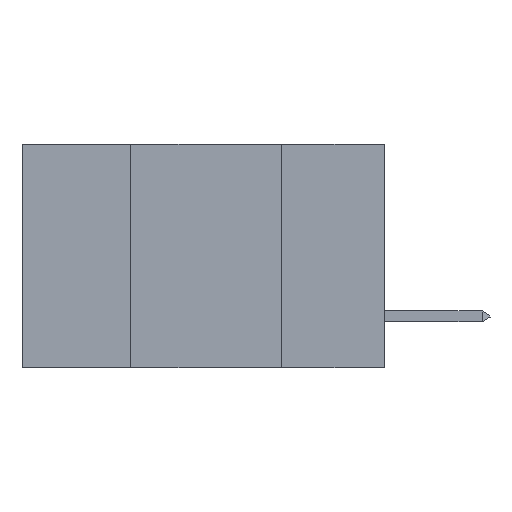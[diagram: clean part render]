
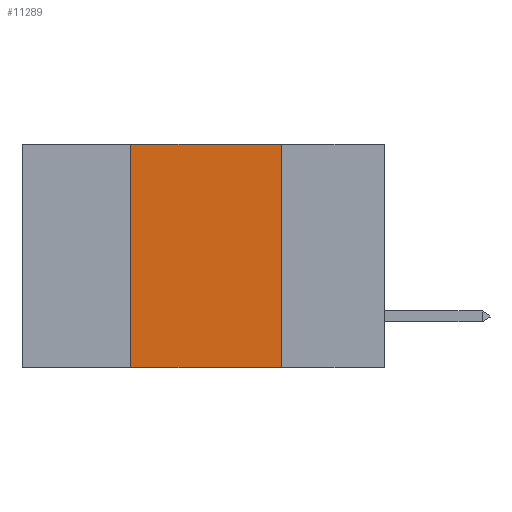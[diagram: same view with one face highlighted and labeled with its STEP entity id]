
A CAD part, left-side view. The second image highlights one B-rep face of the part: STEP entity #11289.
In plain terms, the highlighted planar face has unit normal (-1, 0, 0).
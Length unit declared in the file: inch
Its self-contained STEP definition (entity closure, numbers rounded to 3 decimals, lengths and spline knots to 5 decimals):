
#246 = CARTESIAN_POINT ( 'NONE',  ( 0., 0.6, -0.37 ) ) ;
#308 = DIRECTION ( 'NONE',  ( 0., -1., 0. ) ) ;
#869 = CARTESIAN_POINT ( 'NONE',  ( 0., 0.6, 0. ) ) ;
#902 = VECTOR ( 'NONE', #6013, 39.37008 ) ;
#1194 = CARTESIAN_POINT ( 'NONE',  ( 0., 0.17, 0. ) ) ;
#1370 = LINE ( 'NONE', #4481, #902 ) ;
#2020 = VECTOR ( 'NONE', #308, 39.37008 ) ;
#2426 = DIRECTION ( 'NONE',  ( 0., -1., 0. ) ) ;
#3811 = CARTESIAN_POINT ( 'NONE',  ( 0., 0.6, 0. ) ) ;
#4481 = CARTESIAN_POINT ( 'NONE',  ( 0., 0.42, 0. ) ) ;
#4697 = DIRECTION ( 'NONE',  ( 0., 0., -1. ) ) ;
#4930 = CARTESIAN_POINT ( 'NONE',  ( 0., 0.17, -0.37 ) ) ;
#5173 = VERTEX_POINT ( 'NONE', #4930 ) ;
#5289 = PLANE ( 'NONE',  #15964 ) ;
#5354 = DIRECTION ( 'NONE',  ( 0., 0., -1. ) ) ;
#5594 = LINE ( 'NONE', #246, #2020 ) ;
#6013 = DIRECTION ( 'NONE',  ( 0., 0., 1. ) ) ;
#6210 = VERTEX_POINT ( 'NONE', #16671 ) ;
#6997 = ORIENTED_EDGE ( 'NONE', *, *, #18526, .F. ) ;
#8003 = CARTESIAN_POINT ( 'NONE',  ( 0., 0.42, 0. ) ) ;
#9932 = EDGE_CURVE ( 'NONE', #18668, #5173, #13942, .T. ) ;
#10532 = ORIENTED_EDGE ( 'NONE', *, *, #9932, .F. ) ;
#10671 = VECTOR ( 'NONE', #4697, 39.37008 ) ;
#11003 = ORIENTED_EDGE ( 'NONE', *, *, #12918, .F. ) ;
#11172 = LINE ( 'NONE', #869, #15157 ) ;
#11289 = ADVANCED_FACE ( 'NONE', ( #17158 ), #5289, .F. ) ;
#11432 = EDGE_LOOP ( 'NONE', ( #10532, #6997, #11003, #11442 ) ) ;
#11442 = ORIENTED_EDGE ( 'NONE', *, *, #15940, .T. ) ;
#12174 = CARTESIAN_POINT ( 'NONE',  ( 0., 0.17, 0. ) ) ;
#12918 = EDGE_CURVE ( 'NONE', #6210, #14150, #1370, .T. ) ;
#13942 = LINE ( 'NONE', #12174, #10671 ) ;
#14150 = VERTEX_POINT ( 'NONE', #8003 ) ;
#14339 = DIRECTION ( 'NONE',  ( 1., 0., 0. ) ) ;
#15157 = VECTOR ( 'NONE', #2426, 39.37008 ) ;
#15940 = EDGE_CURVE ( 'NONE', #6210, #5173, #5594, .T. ) ;
#15964 = AXIS2_PLACEMENT_3D ( 'NONE', #3811, #14339, #5354 ) ;
#16671 = CARTESIAN_POINT ( 'NONE',  ( 0., 0.42, -0.37 ) ) ;
#17158 = FACE_OUTER_BOUND ( 'NONE', #11432, .T. ) ;
#18526 = EDGE_CURVE ( 'NONE', #14150, #18668, #11172, .T. ) ;
#18668 = VERTEX_POINT ( 'NONE', #1194 ) ;
